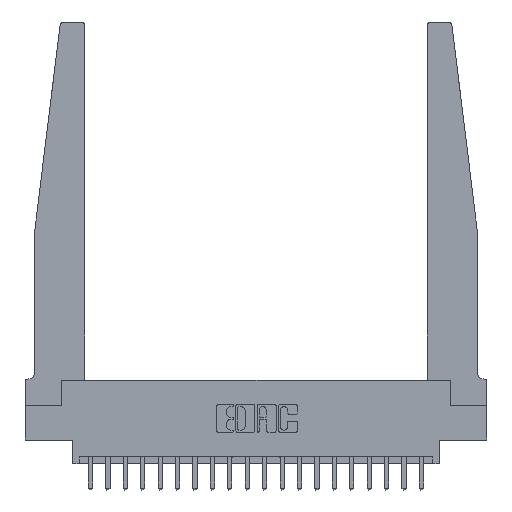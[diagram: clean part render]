
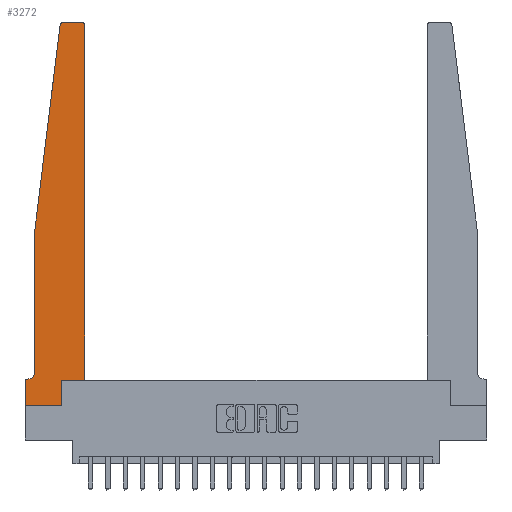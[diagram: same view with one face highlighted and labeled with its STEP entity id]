
A CAD part, top view. The second image highlights one B-rep face of the part: STEP entity #3272.
In plain terms, the highlighted planar face has unit normal (0, 0, 1).
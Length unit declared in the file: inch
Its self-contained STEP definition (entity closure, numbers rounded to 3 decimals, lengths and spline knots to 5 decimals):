
#276 = VERTEX_POINT ( 'NONE', #2547 ) ;
#747 = ORIENTED_EDGE ( 'NONE', *, *, #16242, .T. ) ;
#777 = VERTEX_POINT ( 'NONE', #1332 ) ;
#1053 = LINE ( 'NONE', #11240, #17821 ) ;
#1332 = CARTESIAN_POINT ( 'NONE',  ( 0., 0., 0.37 ) ) ;
#1432 = VERTEX_POINT ( 'NONE', #21006 ) ;
#1733 = AXIS2_PLACEMENT_3D ( 'NONE', #2358, #13698, #4000 ) ;
#1844 = CIRCLE ( 'NONE', #8751, 0.03 ) ;
#1955 = EDGE_CURVE ( 'NONE', #20460, #1432, #14711, .T. ) ;
#2131 = EDGE_LOOP ( 'NONE', ( #18343, #12018, #11697, #12197, #9876, #7406, #3909, #13424, #12004, #15432, #17770, #747 ) ) ;
#2358 = CARTESIAN_POINT ( 'NONE',  ( 0.015, 0.2375, 0.37 ) ) ;
#2504 = EDGE_CURVE ( 'NONE', #1432, #10446, #12610, .T. ) ;
#2547 = CARTESIAN_POINT ( 'NONE',  ( 0.27653, 2.75, 0.37 ) ) ;
#2876 = LINE ( 'NONE', #14956, #7158 ) ;
#2962 = DIRECTION ( 'NONE',  ( 1., 0., 0. ) ) ;
#3110 = DIRECTION ( 'NONE',  ( 1., 0., 0. ) ) ;
#3126 = DIRECTION ( 'NONE',  ( 0., 0., 1. ) ) ;
#3155 = CARTESIAN_POINT ( 'NONE',  ( 0., 0.1875, 0.37 ) ) ;
#3185 = VECTOR ( 'NONE', #9132, 39.37008 ) ;
#3188 = PLANE ( 'NONE',  #11415 ) ;
#3272 = ADVANCED_FACE ( 'NONE', ( #12297 ), #3188, .T. ) ;
#3613 = DIRECTION ( 'NONE',  ( -1., 0., 0. ) ) ;
#3909 = ORIENTED_EDGE ( 'NONE', *, *, #19528, .T. ) ;
#3953 = DIRECTION ( 'NONE',  ( 0., 0., 1. ) ) ;
#4000 = DIRECTION ( 'NONE',  ( -1., 0., 0. ) ) ;
#4296 = EDGE_CURVE ( 'NONE', #13927, #8122, #7475, .T. ) ;
#4421 = VERTEX_POINT ( 'NONE', #6156 ) ;
#4638 = VECTOR ( 'NONE', #7286, 39.37008 ) ;
#4734 = VERTEX_POINT ( 'NONE', #15245 ) ;
#5041 = CARTESIAN_POINT ( 'NONE',  ( 0.425, 0.18, 0.37 ) ) ;
#5141 = LINE ( 'NONE', #5652, #4638 ) ;
#5652 = CARTESIAN_POINT ( 'NONE',  ( 0.065, 0.1875, 0.37 ) ) ;
#5872 = EDGE_CURVE ( 'NONE', #10446, #11433, #15197, .T. ) ;
#5879 = CARTESIAN_POINT ( 'NONE',  ( 0.425, 0.18, 0.37 ) ) ;
#6156 = CARTESIAN_POINT ( 'NONE',  ( 0.2605, 0.18, 0.37 ) ) ;
#6345 = LINE ( 'NONE', #7041, #18324 ) ;
#7041 = CARTESIAN_POINT ( 'NONE',  ( 0., 0., 0.37 ) ) ;
#7158 = VECTOR ( 'NONE', #3613, 39.37008 ) ;
#7286 = DIRECTION ( 'NONE',  ( -1., 0., 0. ) ) ;
#7406 = ORIENTED_EDGE ( 'NONE', *, *, #18944, .T. ) ;
#7475 = LINE ( 'NONE', #5879, #3185 ) ;
#7672 = VECTOR ( 'NONE', #9892, 39.37008 ) ;
#8122 = VERTEX_POINT ( 'NONE', #11834 ) ;
#8335 = VECTOR ( 'NONE', #2962, 39.37008 ) ;
#8564 = CARTESIAN_POINT ( 'NONE',  ( 0.2605, 0., 0.37 ) ) ;
#8751 = AXIS2_PLACEMENT_3D ( 'NONE', #18784, #9004, #20396 ) ;
#9004 = DIRECTION ( 'NONE',  ( 0., 0., 1. ) ) ;
#9132 = DIRECTION ( 'NONE',  ( 0., 1., 0. ) ) ;
#9180 = CARTESIAN_POINT ( 'NONE',  ( 0.015, 0.1875, 0.37 ) ) ;
#9352 = EDGE_CURVE ( 'NONE', #4421, #13927, #20663, .T. ) ;
#9412 = EDGE_CURVE ( 'NONE', #16072, #276, #2876, .T. ) ;
#9597 = CARTESIAN_POINT ( 'NONE',  ( 0.425, 0.18, 0.37 ) ) ;
#9876 = ORIENTED_EDGE ( 'NONE', *, *, #5872, .T. ) ;
#9892 = DIRECTION ( 'NONE',  ( 1., 0., 0. ) ) ;
#10066 = DIRECTION ( 'NONE',  ( 0., -1., 0. ) ) ;
#10084 = CARTESIAN_POINT ( 'NONE',  ( 0.065, 1.25, 0.37 ) ) ;
#10315 = EDGE_CURVE ( 'NONE', #13005, #4421, #1053, .T. ) ;
#10446 = VERTEX_POINT ( 'NONE', #16553 ) ;
#11148 = CARTESIAN_POINT ( 'NONE',  ( 0.24675, 2.72367, 0.37 ) ) ;
#11240 = CARTESIAN_POINT ( 'NONE',  ( 0.2605, 0.18, 0.37 ) ) ;
#11415 = AXIS2_PLACEMENT_3D ( 'NONE', #3155, #3126, #3110 ) ;
#11433 = VERTEX_POINT ( 'NONE', #9180 ) ;
#11697 = ORIENTED_EDGE ( 'NONE', *, *, #1955, .T. ) ;
#11834 = CARTESIAN_POINT ( 'NONE',  ( 0.425, 2.72, 0.37 ) ) ;
#12004 = ORIENTED_EDGE ( 'NONE', *, *, #10315, .T. ) ;
#12018 = ORIENTED_EDGE ( 'NONE', *, *, #17728, .T. ) ;
#12197 = ORIENTED_EDGE ( 'NONE', *, *, #2504, .T. ) ;
#12297 = FACE_OUTER_BOUND ( 'NONE', #2131, .T. ) ;
#12610 = LINE ( 'NONE', #10084, #16953 ) ;
#13005 = VERTEX_POINT ( 'NONE', #8564 ) ;
#13424 = ORIENTED_EDGE ( 'NONE', *, *, #17872, .T. ) ;
#13659 = CARTESIAN_POINT ( 'NONE',  ( 0.27653, 2.72, 0.37 ) ) ;
#13698 = DIRECTION ( 'NONE',  ( 0., 0., -1. ) ) ;
#13927 = VERTEX_POINT ( 'NONE', #9597 ) ;
#14300 = CARTESIAN_POINT ( 'NONE',  ( 0., 0., 0.37 ) ) ;
#14711 = LINE ( 'NONE', #15579, #18515 ) ;
#14782 = AXIS2_PLACEMENT_3D ( 'NONE', #13659, #3953, #15301 ) ;
#14956 = CARTESIAN_POINT ( 'NONE',  ( 0.25, 2.75, 0.37 ) ) ;
#15057 = CARTESIAN_POINT ( 'NONE',  ( 0.395, 2.75, 0.37 ) ) ;
#15197 = CIRCLE ( 'NONE', #1733, 0.05 ) ;
#15245 = CARTESIAN_POINT ( 'NONE',  ( 0., 0.1875, 0.37 ) ) ;
#15301 = DIRECTION ( 'NONE',  ( 1., 0., 0. ) ) ;
#15432 = ORIENTED_EDGE ( 'NONE', *, *, #9352, .T. ) ;
#15550 = DIRECTION ( 'NONE',  ( -0.122, -0.992, 0. ) ) ;
#15579 = CARTESIAN_POINT ( 'NONE',  ( 0.065, 1.25, 0.37 ) ) ;
#16072 = VERTEX_POINT ( 'NONE', #15057 ) ;
#16242 = EDGE_CURVE ( 'NONE', #8122, #16072, #1844, .T. ) ;
#16553 = CARTESIAN_POINT ( 'NONE',  ( 0.065, 0.2375, 0.37 ) ) ;
#16953 = VECTOR ( 'NONE', #10066, 39.37008 ) ;
#17002 = LINE ( 'NONE', #14300, #8335 ) ;
#17728 = EDGE_CURVE ( 'NONE', #276, #20460, #19069, .T. ) ;
#17770 = ORIENTED_EDGE ( 'NONE', *, *, #4296, .T. ) ;
#17821 = VECTOR ( 'NONE', #17851, 39.37008 ) ;
#17851 = DIRECTION ( 'NONE',  ( 0., 1., 0. ) ) ;
#17872 = EDGE_CURVE ( 'NONE', #777, #13005, #17002, .T. ) ;
#18324 = VECTOR ( 'NONE', #20070, 39.37008 ) ;
#18343 = ORIENTED_EDGE ( 'NONE', *, *, #9412, .T. ) ;
#18515 = VECTOR ( 'NONE', #15550, 39.37008 ) ;
#18784 = CARTESIAN_POINT ( 'NONE',  ( 0.395, 2.72, 0.37 ) ) ;
#18944 = EDGE_CURVE ( 'NONE', #11433, #4734, #5141, .T. ) ;
#19069 = CIRCLE ( 'NONE', #14782, 0.03 ) ;
#19528 = EDGE_CURVE ( 'NONE', #4734, #777, #6345, .T. ) ;
#20070 = DIRECTION ( 'NONE',  ( 0., -1., 0. ) ) ;
#20396 = DIRECTION ( 'NONE',  ( 1., 0., 0. ) ) ;
#20460 = VERTEX_POINT ( 'NONE', #11148 ) ;
#20663 = LINE ( 'NONE', #5041, #7672 ) ;
#21006 = CARTESIAN_POINT ( 'NONE',  ( 0.065, 1.25, 0.37 ) ) ;
